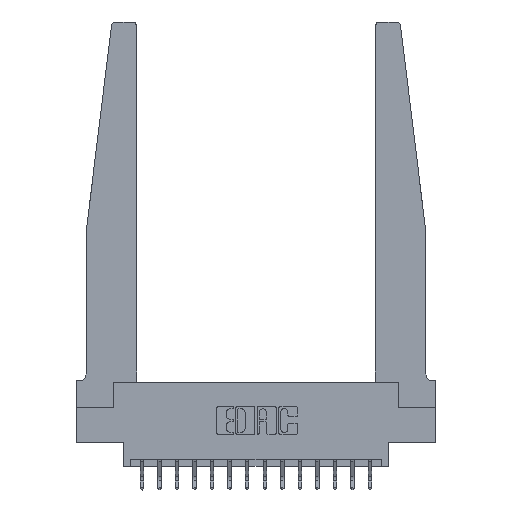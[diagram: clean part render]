
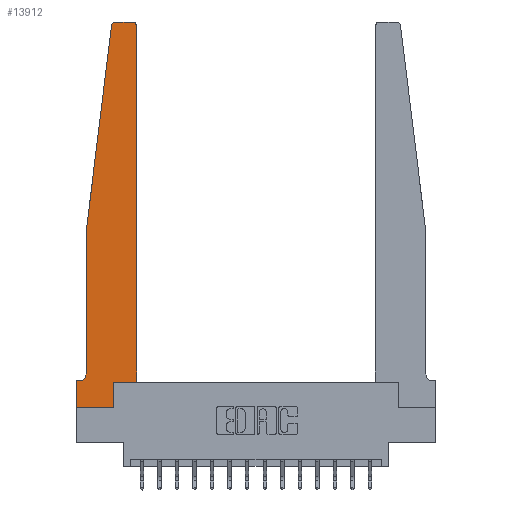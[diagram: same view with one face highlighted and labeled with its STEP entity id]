
A CAD part, top view. The second image highlights one B-rep face of the part: STEP entity #13912.
In plain terms, the highlighted planar face has unit normal (0, 0, 1).
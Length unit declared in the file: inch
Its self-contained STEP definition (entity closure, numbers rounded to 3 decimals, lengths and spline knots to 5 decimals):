
#209 = CIRCLE ( 'NONE', #15868, 0.03 ) ;
#221 = CARTESIAN_POINT ( 'NONE',  ( 0., 0., 0.37 ) ) ;
#395 = VECTOR ( 'NONE', #4643, 39.37008 ) ;
#499 = VERTEX_POINT ( 'NONE', #5510 ) ;
#668 = DIRECTION ( 'NONE',  ( 0., 0., 1. ) ) ;
#744 = VERTEX_POINT ( 'NONE', #3516 ) ;
#1064 = LINE ( 'NONE', #221, #11717 ) ;
#1188 = EDGE_CURVE ( 'NONE', #4038, #2404, #2378, .T. ) ;
#1574 = EDGE_CURVE ( 'NONE', #2404, #1745, #4088, .T. ) ;
#1665 = CARTESIAN_POINT ( 'NONE',  ( 0.425, 0.18, 0.37 ) ) ;
#1745 = VERTEX_POINT ( 'NONE', #3020 ) ;
#1901 = LINE ( 'NONE', #11205, #6040 ) ;
#1906 = ORIENTED_EDGE ( 'NONE', *, *, #9437, .T. ) ;
#2378 = LINE ( 'NONE', #1665, #6510 ) ;
#2404 = VERTEX_POINT ( 'NONE', #16882 ) ;
#2448 = EDGE_CURVE ( 'NONE', #499, #744, #5807, .T. ) ;
#2777 = ORIENTED_EDGE ( 'NONE', *, *, #6591, .T. ) ;
#2911 = AXIS2_PLACEMENT_3D ( 'NONE', #17208, #3314, #13034 ) ;
#2968 = VECTOR ( 'NONE', #11426, 39.37008 ) ;
#3020 = CARTESIAN_POINT ( 'NONE',  ( 0.425, 2.72, 0.37 ) ) ;
#3073 = EDGE_CURVE ( 'NONE', #1745, #5710, #10811, .T. ) ;
#3280 = EDGE_CURVE ( 'NONE', #17250, #4038, #12316, .T. ) ;
#3314 = DIRECTION ( 'NONE',  ( 0., 0., 1. ) ) ;
#3516 = CARTESIAN_POINT ( 'NONE',  ( 0., 0.1875, 0.37 ) ) ;
#3639 = ORIENTED_EDGE ( 'NONE', *, *, #3280, .T. ) ;
#4038 = VERTEX_POINT ( 'NONE', #15539 ) ;
#4088 = LINE ( 'NONE', #16582, #395 ) ;
#4155 = CIRCLE ( 'NONE', #13696, 0.05 ) ;
#4280 = DIRECTION ( 'NONE',  ( 0., -1., 0. ) ) ;
#4643 = DIRECTION ( 'NONE',  ( 0., 1., 0. ) ) ;
#4721 = CARTESIAN_POINT ( 'NONE',  ( 0.065, 0.2375, 0.37 ) ) ;
#4733 = ORIENTED_EDGE ( 'NONE', *, *, #12400, .T. ) ;
#4972 = CARTESIAN_POINT ( 'NONE',  ( 0.27653, 2.75, 0.37 ) ) ;
#5018 = CARTESIAN_POINT ( 'NONE',  ( 0.015, 0.2375, 0.37 ) ) ;
#5312 = CARTESIAN_POINT ( 'NONE',  ( 0.2605, 0.18, 0.37 ) ) ;
#5510 = CARTESIAN_POINT ( 'NONE',  ( 0.015, 0.1875, 0.37 ) ) ;
#5677 = EDGE_CURVE ( 'NONE', #7652, #10140, #9393, .T. ) ;
#5710 = VERTEX_POINT ( 'NONE', #16993 ) ;
#5807 = LINE ( 'NONE', #5862, #2968 ) ;
#5862 = CARTESIAN_POINT ( 'NONE',  ( 0.065, 0.1875, 0.37 ) ) ;
#5998 = LINE ( 'NONE', #13395, #8794 ) ;
#6040 = VECTOR ( 'NONE', #4280, 39.37008 ) ;
#6202 = CARTESIAN_POINT ( 'NONE',  ( 0.27653, 2.72, 0.37 ) ) ;
#6410 = DIRECTION ( 'NONE',  ( -1., 0., 0. ) ) ;
#6465 = ORIENTED_EDGE ( 'NONE', *, *, #1574, .T. ) ;
#6482 = DIRECTION ( 'NONE',  ( -1., 0., 0. ) ) ;
#6510 = VECTOR ( 'NONE', #14979, 39.37008 ) ;
#6529 = VERTEX_POINT ( 'NONE', #4972 ) ;
#6591 = EDGE_CURVE ( 'NONE', #5710, #6529, #5998, .T. ) ;
#7166 = CARTESIAN_POINT ( 'NONE',  ( 0.065, 1.25, 0.37 ) ) ;
#7586 = DIRECTION ( 'NONE',  ( 1., 0., 0. ) ) ;
#7652 = VERTEX_POINT ( 'NONE', #10067 ) ;
#7745 = CARTESIAN_POINT ( 'NONE',  ( 0.2605, 0., 0.37 ) ) ;
#8122 = AXIS2_PLACEMENT_3D ( 'NONE', #8974, #668, #10374 ) ;
#8174 = VECTOR ( 'NONE', #16451, 39.37008 ) ;
#8402 = ORIENTED_EDGE ( 'NONE', *, *, #2448, .T. ) ;
#8511 = DIRECTION ( 'NONE',  ( 1., 0., 0. ) ) ;
#8538 = DIRECTION ( 'NONE',  ( 0., -1., 0. ) ) ;
#8794 = VECTOR ( 'NONE', #6482, 39.37008 ) ;
#8817 = PLANE ( 'NONE',  #2911 ) ;
#8837 = ORIENTED_EDGE ( 'NONE', *, *, #9092, .T. ) ;
#8974 = CARTESIAN_POINT ( 'NONE',  ( 0.395, 2.72, 0.37 ) ) ;
#9092 = EDGE_CURVE ( 'NONE', #10140, #499, #4155, .T. ) ;
#9393 = LINE ( 'NONE', #7166, #12660 ) ;
#9437 = EDGE_CURVE ( 'NONE', #10859, #7652, #13725, .T. ) ;
#10067 = CARTESIAN_POINT ( 'NONE',  ( 0.065, 1.25, 0.37 ) ) ;
#10125 = ORIENTED_EDGE ( 'NONE', *, *, #1188, .T. ) ;
#10140 = VERTEX_POINT ( 'NONE', #4721 ) ;
#10374 = DIRECTION ( 'NONE',  ( 1., 0., 0. ) ) ;
#10386 = DIRECTION ( 'NONE',  ( -0.122, -0.992, 0. ) ) ;
#10540 = EDGE_LOOP ( 'NONE', ( #2777, #13423, #1906, #16309, #8837, #8402, #4733, #14740, #3639, #10125, #6465, #16706 ) ) ;
#10811 = CIRCLE ( 'NONE', #8122, 0.03 ) ;
#10859 = VERTEX_POINT ( 'NONE', #17323 ) ;
#11205 = CARTESIAN_POINT ( 'NONE',  ( 0., 0., 0.37 ) ) ;
#11426 = DIRECTION ( 'NONE',  ( -1., 0., 0. ) ) ;
#11717 = VECTOR ( 'NONE', #8511, 39.37008 ) ;
#11739 = CARTESIAN_POINT ( 'NONE',  ( 0.065, 1.25, 0.37 ) ) ;
#12316 = LINE ( 'NONE', #5312, #8174 ) ;
#12400 = EDGE_CURVE ( 'NONE', #744, #13037, #1901, .T. ) ;
#12660 = VECTOR ( 'NONE', #8538, 39.37008 ) ;
#13034 = DIRECTION ( 'NONE',  ( 1., 0., 0. ) ) ;
#13037 = VERTEX_POINT ( 'NONE', #13855 ) ;
#13395 = CARTESIAN_POINT ( 'NONE',  ( 0.25, 2.75, 0.37 ) ) ;
#13423 = ORIENTED_EDGE ( 'NONE', *, *, #15169, .T. ) ;
#13696 = AXIS2_PLACEMENT_3D ( 'NONE', #5018, #14746, #6410 ) ;
#13725 = LINE ( 'NONE', #11739, #17019 ) ;
#13855 = CARTESIAN_POINT ( 'NONE',  ( 0., 0., 0.37 ) ) ;
#13912 = ADVANCED_FACE ( 'NONE', ( #14839 ), #8817, .T. ) ;
#14740 = ORIENTED_EDGE ( 'NONE', *, *, #15646, .T. ) ;
#14746 = DIRECTION ( 'NONE',  ( 0., 0., -1. ) ) ;
#14839 = FACE_OUTER_BOUND ( 'NONE', #10540, .T. ) ;
#14979 = DIRECTION ( 'NONE',  ( 1., 0., 0. ) ) ;
#15169 = EDGE_CURVE ( 'NONE', #6529, #10859, #209, .T. ) ;
#15539 = CARTESIAN_POINT ( 'NONE',  ( 0.2605, 0.18, 0.37 ) ) ;
#15646 = EDGE_CURVE ( 'NONE', #13037, #17250, #1064, .T. ) ;
#15868 = AXIS2_PLACEMENT_3D ( 'NONE', #6202, #15945, #7586 ) ;
#15945 = DIRECTION ( 'NONE',  ( 0., 0., 1. ) ) ;
#16309 = ORIENTED_EDGE ( 'NONE', *, *, #5677, .T. ) ;
#16451 = DIRECTION ( 'NONE',  ( 0., 1., 0. ) ) ;
#16582 = CARTESIAN_POINT ( 'NONE',  ( 0.425, 0.18, 0.37 ) ) ;
#16706 = ORIENTED_EDGE ( 'NONE', *, *, #3073, .T. ) ;
#16882 = CARTESIAN_POINT ( 'NONE',  ( 0.425, 0.18, 0.37 ) ) ;
#16993 = CARTESIAN_POINT ( 'NONE',  ( 0.395, 2.75, 0.37 ) ) ;
#17019 = VECTOR ( 'NONE', #10386, 39.37008 ) ;
#17208 = CARTESIAN_POINT ( 'NONE',  ( 0., 0.1875, 0.37 ) ) ;
#17250 = VERTEX_POINT ( 'NONE', #7745 ) ;
#17323 = CARTESIAN_POINT ( 'NONE',  ( 0.24675, 2.72367, 0.37 ) ) ;
